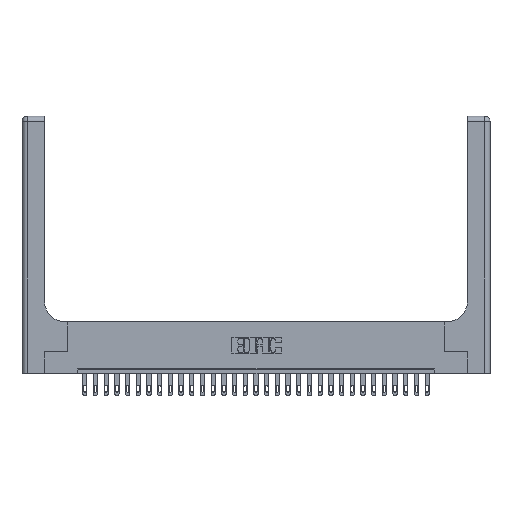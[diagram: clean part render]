
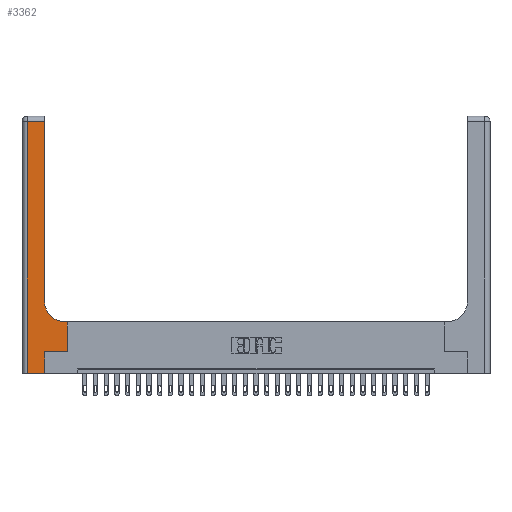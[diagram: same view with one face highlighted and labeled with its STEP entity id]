
A CAD part, top view. The second image highlights one B-rep face of the part: STEP entity #3362.
In plain terms, the highlighted planar face has unit normal (0, 0, 1).
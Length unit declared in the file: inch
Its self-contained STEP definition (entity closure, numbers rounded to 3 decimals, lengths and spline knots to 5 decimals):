
#397 = PLANE ( 'NONE',  #17783 ) ;
#1431 = VECTOR ( 'NONE', #22674, 39.37008 ) ;
#1446 = CARTESIAN_POINT ( 'NONE',  ( 0.265, 0.25, 0.37 ) ) ;
#1870 = CARTESIAN_POINT ( 'NONE',  ( 0.265, 0., 0.37 ) ) ;
#2133 = LINE ( 'NONE', #10725, #5015 ) ;
#2244 = VERTEX_POINT ( 'NONE', #2617 ) ;
#2417 = EDGE_CURVE ( 'NONE', #4759, #20482, #2133, .T. ) ;
#2481 = FACE_OUTER_BOUND ( 'NONE', #27073, .T. ) ;
#2617 = CARTESIAN_POINT ( 'NONE',  ( 0.528, 0.6, 0.37 ) ) ;
#3271 = DIRECTION ( 'NONE',  ( 0., 1., 0. ) ) ;
#3362 = ADVANCED_FACE ( 'NONE', ( #2481 ), #397, .F. ) ;
#4116 = ORIENTED_EDGE ( 'NONE', *, *, #19883, .T. ) ;
#4320 = VECTOR ( 'NONE', #20357, 39.37008 ) ;
#4370 = DIRECTION ( 'NONE',  ( 1., 0., 0. ) ) ;
#4403 = CARTESIAN_POINT ( 'NONE',  ( 0.26, 2.94, 0.37 ) ) ;
#4737 = EDGE_CURVE ( 'NONE', #6904, #25589, #5357, .T. ) ;
#4759 = VERTEX_POINT ( 'NONE', #1446 ) ;
#4858 = EDGE_CURVE ( 'NONE', #19971, #13170, #5898, .T. ) ;
#4875 = CIRCLE ( 'NONE', #25090, 0.25 ) ;
#5015 = VECTOR ( 'NONE', #4370, 39.37008 ) ;
#5357 = LINE ( 'NONE', #24341, #10363 ) ;
#5380 = CARTESIAN_POINT ( 'NONE',  ( 0.06, 3., 0.37 ) ) ;
#5898 = LINE ( 'NONE', #11988, #1431 ) ;
#6131 = CARTESIAN_POINT ( 'NONE',  ( 0.528, 0.25, 0.37 ) ) ;
#6175 = LINE ( 'NONE', #12543, #17808 ) ;
#6369 = CARTESIAN_POINT ( 'NONE',  ( 0.06, 2.94, 0.37 ) ) ;
#6777 = DIRECTION ( 'NONE',  ( -1., 0., 0. ) ) ;
#6904 = VERTEX_POINT ( 'NONE', #17827 ) ;
#7191 = DIRECTION ( 'NONE',  ( -1., 0., 0. ) ) ;
#7519 = VERTEX_POINT ( 'NONE', #6369 ) ;
#7602 = LINE ( 'NONE', #17788, #11040 ) ;
#8017 = EDGE_CURVE ( 'NONE', #25589, #7519, #19465, .T. ) ;
#8690 = VERTEX_POINT ( 'NONE', #20489 ) ;
#8728 = ORIENTED_EDGE ( 'NONE', *, *, #14466, .T. ) ;
#8843 = CARTESIAN_POINT ( 'NONE',  ( 0., 3., 0.37 ) ) ;
#9611 = CARTESIAN_POINT ( 'NONE',  ( 0.528, 0.25, 0.37 ) ) ;
#10363 = VECTOR ( 'NONE', #3271, 39.37008 ) ;
#10407 = VECTOR ( 'NONE', #22294, 39.37008 ) ;
#10465 = VECTOR ( 'NONE', #15326, 39.37008 ) ;
#10725 = CARTESIAN_POINT ( 'NONE',  ( 0.265, 0.25, 0.37 ) ) ;
#10815 = ORIENTED_EDGE ( 'NONE', *, *, #22360, .T. ) ;
#11040 = VECTOR ( 'NONE', #7191, 39.37008 ) ;
#11278 = DIRECTION ( 'NONE',  ( 1., 0., 0. ) ) ;
#11445 = ORIENTED_EDGE ( 'NONE', *, *, #24464, .T. ) ;
#11598 = LINE ( 'NONE', #5380, #10407 ) ;
#11988 = CARTESIAN_POINT ( 'NONE',  ( 0., 0., 0.37 ) ) ;
#12543 = CARTESIAN_POINT ( 'NONE',  ( 0.265, 0., 0.37 ) ) ;
#13170 = VERTEX_POINT ( 'NONE', #1870 ) ;
#14466 = EDGE_CURVE ( 'NONE', #13170, #4759, #6175, .T. ) ;
#15225 = ORIENTED_EDGE ( 'NONE', *, *, #4737, .T. ) ;
#15326 = DIRECTION ( 'NONE',  ( -1., 0., 0. ) ) ;
#15979 = EDGE_CURVE ( 'NONE', #7519, #19971, #11598, .T. ) ;
#16829 = ORIENTED_EDGE ( 'NONE', *, *, #15979, .T. ) ;
#16926 = DIRECTION ( 'NONE',  ( 0., 1., 0. ) ) ;
#17123 = CARTESIAN_POINT ( 'NONE',  ( 0., 2.94, 0.37 ) ) ;
#17245 = DIRECTION ( 'NONE',  ( 0., 0., -1. ) ) ;
#17307 = ORIENTED_EDGE ( 'NONE', *, *, #2417, .T. ) ;
#17783 = AXIS2_PLACEMENT_3D ( 'NONE', #8843, #17245, #6777 ) ;
#17788 = CARTESIAN_POINT ( 'NONE',  ( 0.26, 0.6, 0.37 ) ) ;
#17808 = VECTOR ( 'NONE', #16926, 39.37008 ) ;
#17827 = CARTESIAN_POINT ( 'NONE',  ( 0.26, 0.85, 0.37 ) ) ;
#17989 = CARTESIAN_POINT ( 'NONE',  ( 0.51, 0.85, 0.37 ) ) ;
#18658 = ORIENTED_EDGE ( 'NONE', *, *, #4858, .T. ) ;
#19465 = LINE ( 'NONE', #17123, #10465 ) ;
#19665 = DIRECTION ( 'NONE',  ( 0., 0., -1. ) ) ;
#19883 = EDGE_CURVE ( 'NONE', #20482, #2244, #23930, .T. ) ;
#19971 = VERTEX_POINT ( 'NONE', #26389 ) ;
#20357 = DIRECTION ( 'NONE',  ( 0., 1., 0. ) ) ;
#20482 = VERTEX_POINT ( 'NONE', #6131 ) ;
#20489 = CARTESIAN_POINT ( 'NONE',  ( 0.51, 0.6, 0.37 ) ) ;
#21918 = ORIENTED_EDGE ( 'NONE', *, *, #8017, .T. ) ;
#22294 = DIRECTION ( 'NONE',  ( 0., -1., 0. ) ) ;
#22360 = EDGE_CURVE ( 'NONE', #2244, #8690, #7602, .T. ) ;
#22674 = DIRECTION ( 'NONE',  ( 1., 0., 0. ) ) ;
#23930 = LINE ( 'NONE', #9611, #4320 ) ;
#24341 = CARTESIAN_POINT ( 'NONE',  ( 0.26, 3., 0.37 ) ) ;
#24464 = EDGE_CURVE ( 'NONE', #8690, #6904, #4875, .T. ) ;
#25090 = AXIS2_PLACEMENT_3D ( 'NONE', #17989, #19665, #11278 ) ;
#25589 = VERTEX_POINT ( 'NONE', #4403 ) ;
#26389 = CARTESIAN_POINT ( 'NONE',  ( 0.06, 0., 0.37 ) ) ;
#27073 = EDGE_LOOP ( 'NONE', ( #15225, #21918, #16829, #18658, #8728, #17307, #4116, #10815, #11445 ) ) ;
